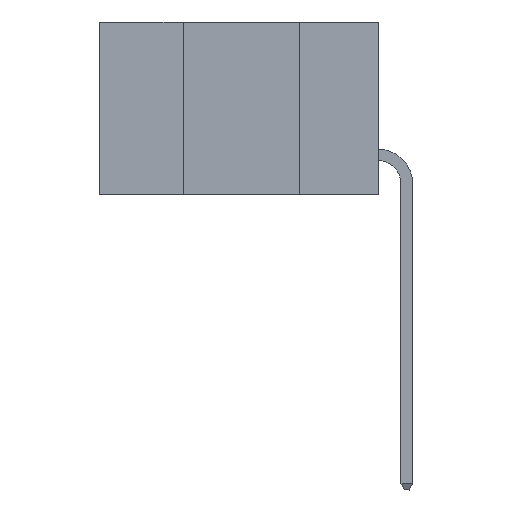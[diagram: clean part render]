
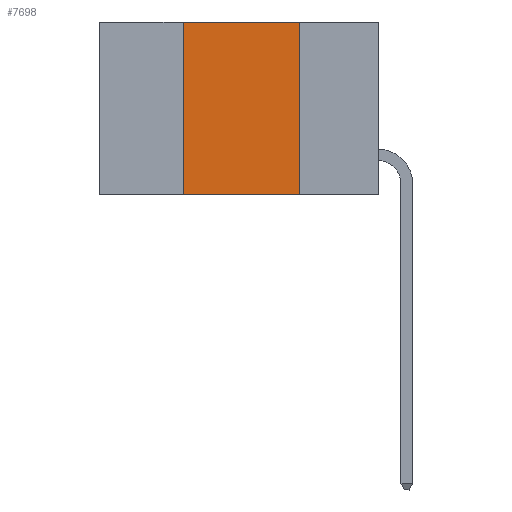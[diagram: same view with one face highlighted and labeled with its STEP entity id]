
A CAD part, left-side view. The second image highlights one B-rep face of the part: STEP entity #7698.
In plain terms, the highlighted planar face has unit normal (-1, 0, 0).
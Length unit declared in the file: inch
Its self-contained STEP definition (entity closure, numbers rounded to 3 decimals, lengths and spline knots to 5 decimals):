
#1424 = CARTESIAN_POINT ( 'NONE',  ( 0., 0.6, 0. ) ) ;
#3218 = VERTEX_POINT ( 'NONE', #29729 ) ;
#4017 = FACE_OUTER_BOUND ( 'NONE', #11400, .T. ) ;
#4773 = ORIENTED_EDGE ( 'NONE', *, *, #10609, .F. ) ;
#5970 = VERTEX_POINT ( 'NONE', #11662 ) ;
#6891 = DIRECTION ( 'NONE',  ( 0., 0., 1. ) ) ;
#7698 = ADVANCED_FACE ( 'NONE', ( #4017 ), #27288, .F. ) ;
#8266 = ORIENTED_EDGE ( 'NONE', *, *, #12537, .T. ) ;
#8327 = LINE ( 'NONE', #1424, #22890 ) ;
#8533 = DIRECTION ( 'NONE',  ( 0., -1., 0. ) ) ;
#8884 = VERTEX_POINT ( 'NONE', #25320 ) ;
#9215 = DIRECTION ( 'NONE',  ( 0., -1., 0. ) ) ;
#9317 = CARTESIAN_POINT ( 'NONE',  ( 0., 0.6, 0. ) ) ;
#9609 = VECTOR ( 'NONE', #9630, 39.37008 ) ;
#9630 = DIRECTION ( 'NONE',  ( 0., 0., -1. ) ) ;
#10609 = EDGE_CURVE ( 'NONE', #30907, #5970, #26670, .T. ) ;
#10793 = ORIENTED_EDGE ( 'NONE', *, *, #28922, .F. ) ;
#10895 = CARTESIAN_POINT ( 'NONE',  ( 0., 0.6, -0.37 ) ) ;
#11196 = AXIS2_PLACEMENT_3D ( 'NONE', #9317, #22433, #14513 ) ;
#11390 = CARTESIAN_POINT ( 'NONE',  ( 0., 0.42, -0.37 ) ) ;
#11400 = EDGE_LOOP ( 'NONE', ( #10793, #30237, #4773, #8266 ) ) ;
#11662 = CARTESIAN_POINT ( 'NONE',  ( 0., 0.42, 0. ) ) ;
#12537 = EDGE_CURVE ( 'NONE', #30907, #3218, #20058, .T. ) ;
#14513 = DIRECTION ( 'NONE',  ( 0., 0., -1. ) ) ;
#20058 = LINE ( 'NONE', #10895, #32071 ) ;
#21350 = LINE ( 'NONE', #22751, #9609 ) ;
#22353 = CARTESIAN_POINT ( 'NONE',  ( 0., 0.42, 0. ) ) ;
#22433 = DIRECTION ( 'NONE',  ( 1., 0., 0. ) ) ;
#22751 = CARTESIAN_POINT ( 'NONE',  ( 0., 0.17, 0. ) ) ;
#22890 = VECTOR ( 'NONE', #9215, 39.37008 ) ;
#25320 = CARTESIAN_POINT ( 'NONE',  ( 0., 0.17, 0. ) ) ;
#26670 = LINE ( 'NONE', #22353, #29074 ) ;
#27288 = PLANE ( 'NONE',  #11196 ) ;
#28922 = EDGE_CURVE ( 'NONE', #8884, #3218, #21350, .T. ) ;
#29074 = VECTOR ( 'NONE', #6891, 39.37008 ) ;
#29729 = CARTESIAN_POINT ( 'NONE',  ( 0., 0.17, -0.37 ) ) ;
#29977 = EDGE_CURVE ( 'NONE', #5970, #8884, #8327, .T. ) ;
#30237 = ORIENTED_EDGE ( 'NONE', *, *, #29977, .F. ) ;
#30907 = VERTEX_POINT ( 'NONE', #11390 ) ;
#32071 = VECTOR ( 'NONE', #8533, 39.37008 ) ;
